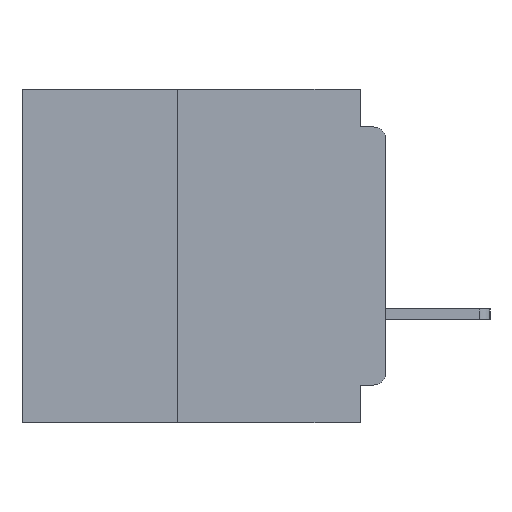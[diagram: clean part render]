
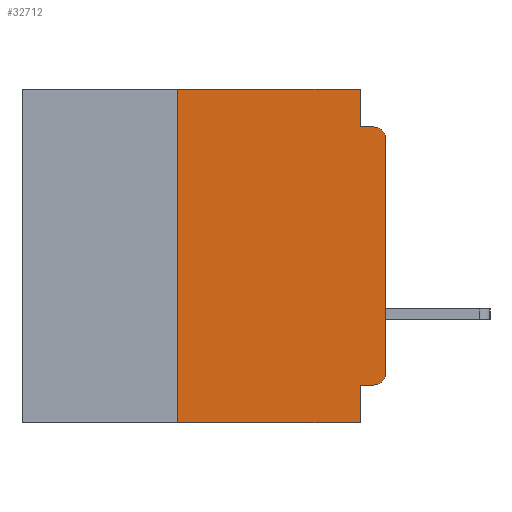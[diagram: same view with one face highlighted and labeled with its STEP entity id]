
A CAD part, left-side view. The second image highlights one B-rep face of the part: STEP entity #32712.
In plain terms, the highlighted planar face has unit normal (-1, 0, 0).
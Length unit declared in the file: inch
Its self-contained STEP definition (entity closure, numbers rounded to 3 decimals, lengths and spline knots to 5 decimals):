
#742 = LINE ( 'NONE', #29667, #42901 ) ;
#1941 = VECTOR ( 'NONE', #19512, 39.37008 ) ;
#3548 = DIRECTION ( 'NONE',  ( 0., 1., 0. ) ) ;
#6197 = ORIENTED_EDGE ( 'NONE', *, *, #39112, .T. ) ;
#7987 = AXIS2_PLACEMENT_3D ( 'NONE', #17794, #46150, #21936 ) ;
#8989 = CARTESIAN_POINT ( 'NONE',  ( 0., 0., 0. ) ) ;
#9048 = CARTESIAN_POINT ( 'NONE',  ( 0., 0.031, -0.045 ) ) ;
#9254 = DIRECTION ( 'NONE',  ( 1., 0., 0. ) ) ;
#9734 = VERTEX_POINT ( 'NONE', #20476 ) ;
#10801 = AXIS2_PLACEMENT_3D ( 'NONE', #39432, #15084, #43482 ) ;
#11377 = VERTEX_POINT ( 'NONE', #9048 ) ;
#12565 = LINE ( 'NONE', #51588, #51837 ) ;
#13140 = VECTOR ( 'NONE', #46904, 39.37008 ) ;
#13155 = DIRECTION ( 'NONE',  ( 0., 0., 1. ) ) ;
#13230 = PLANE ( 'NONE',  #24703 ) ;
#13568 = VERTEX_POINT ( 'NONE', #38144 ) ;
#13709 = ORIENTED_EDGE ( 'NONE', *, *, #46031, .F. ) ;
#14898 = VERTEX_POINT ( 'NONE', #47126 ) ;
#15084 = DIRECTION ( 'NONE',  ( -1., 0., 0. ) ) ;
#15386 = CARTESIAN_POINT ( 'NONE',  ( 0., 0.437, -0.4 ) ) ;
#15509 = EDGE_CURVE ( 'NONE', #13568, #34207, #34827, .T. ) ;
#15622 = EDGE_CURVE ( 'NONE', #34207, #42120, #27241, .T. ) ;
#15964 = CIRCLE ( 'NONE', #7987, 0.015 ) ;
#16896 = CARTESIAN_POINT ( 'NONE',  ( 0., 0.031, -0.4 ) ) ;
#17794 = CARTESIAN_POINT ( 'NONE',  ( 0., 0.015, -0.34 ) ) ;
#17914 = EDGE_CURVE ( 'NONE', #13568, #43147, #23846, .T. ) ;
#18343 = CARTESIAN_POINT ( 'NONE',  ( 0., 0.031, -0.4 ) ) ;
#18580 = CARTESIAN_POINT ( 'NONE',  ( 0., 0.25, -0.4 ) ) ;
#18946 = EDGE_CURVE ( 'NONE', #38450, #43147, #40191, .T. ) ;
#19512 = DIRECTION ( 'NONE',  ( 0., -1., 0. ) ) ;
#20476 = CARTESIAN_POINT ( 'NONE',  ( 0., 0., -0.06 ) ) ;
#21034 = DIRECTION ( 'NONE',  ( 0., 0., -1. ) ) ;
#21538 = FACE_OUTER_BOUND ( 'NONE', #50011, .T. ) ;
#21640 = ORIENTED_EDGE ( 'NONE', *, *, #18946, .F. ) ;
#21936 = DIRECTION ( 'NONE',  ( 0., 0., -1. ) ) ;
#22992 = VECTOR ( 'NONE', #3548, 39.37008 ) ;
#23239 = EDGE_CURVE ( 'NONE', #11377, #14898, #12565, .T. ) ;
#23354 = ORIENTED_EDGE ( 'NONE', *, *, #24759, .F. ) ;
#23600 = CARTESIAN_POINT ( 'NONE',  ( 0., 0.437, 0. ) ) ;
#23846 = LINE ( 'NONE', #15386, #1941 ) ;
#24703 = AXIS2_PLACEMENT_3D ( 'NONE', #25595, #9254, #37783 ) ;
#24759 = EDGE_CURVE ( 'NONE', #42120, #11377, #742, .T. ) ;
#25595 = CARTESIAN_POINT ( 'NONE',  ( 0., 0.437, 0. ) ) ;
#26967 = VERTEX_POINT ( 'NONE', #52429 ) ;
#27241 = LINE ( 'NONE', #23600, #47369 ) ;
#27694 = DIRECTION ( 'NONE',  ( 0., -1., 0. ) ) ;
#28161 = EDGE_CURVE ( 'NONE', #9734, #14898, #46636, .T. ) ;
#29428 = CARTESIAN_POINT ( 'NONE',  ( 0., 0.031, -0.355 ) ) ;
#29667 = CARTESIAN_POINT ( 'NONE',  ( 0., 0.031, 0. ) ) ;
#31478 = ORIENTED_EDGE ( 'NONE', *, *, #17914, .T. ) ;
#31873 = CARTESIAN_POINT ( 'NONE',  ( 0., 0.031, 0. ) ) ;
#32712 = ADVANCED_FACE ( 'NONE', ( #21538 ), #13230, .F. ) ;
#33252 = ORIENTED_EDGE ( 'NONE', *, *, #23239, .F. ) ;
#33271 = VERTEX_POINT ( 'NONE', #50882 ) ;
#34207 = VERTEX_POINT ( 'NONE', #41523 ) ;
#34827 = LINE ( 'NONE', #18580, #13140 ) ;
#35737 = VECTOR ( 'NONE', #13155, 39.37008 ) ;
#36288 = CARTESIAN_POINT ( 'NONE',  ( 0., 0., -0.355 ) ) ;
#36324 = LINE ( 'NONE', #36288, #22992 ) ;
#36413 = VECTOR ( 'NONE', #21034, 39.37008 ) ;
#37783 = DIRECTION ( 'NONE',  ( 0., 0., -1. ) ) ;
#38144 = CARTESIAN_POINT ( 'NONE',  ( 0., 0.25, -0.4 ) ) ;
#38450 = VERTEX_POINT ( 'NONE', #29428 ) ;
#39112 = EDGE_CURVE ( 'NONE', #26967, #9734, #46394, .T. ) ;
#39432 = CARTESIAN_POINT ( 'NONE',  ( 0., 0.015, -0.06 ) ) ;
#40191 = LINE ( 'NONE', #16896, #36413 ) ;
#40944 = ORIENTED_EDGE ( 'NONE', *, *, #45642, .T. ) ;
#41277 = ORIENTED_EDGE ( 'NONE', *, *, #15622, .F. ) ;
#41523 = CARTESIAN_POINT ( 'NONE',  ( 0., 0.25, 0. ) ) ;
#42120 = VERTEX_POINT ( 'NONE', #31873 ) ;
#42901 = VECTOR ( 'NONE', #45627, 39.37008 ) ;
#43147 = VERTEX_POINT ( 'NONE', #18343 ) ;
#43482 = DIRECTION ( 'NONE',  ( 0., 0., -1. ) ) ;
#45627 = DIRECTION ( 'NONE',  ( 0., 0., -1. ) ) ;
#45642 = EDGE_CURVE ( 'NONE', #33271, #26967, #15964, .T. ) ;
#46031 = EDGE_CURVE ( 'NONE', #33271, #38450, #36324, .T. ) ;
#46150 = DIRECTION ( 'NONE',  ( -1., 0., 0. ) ) ;
#46394 = LINE ( 'NONE', #8989, #35737 ) ;
#46636 = CIRCLE ( 'NONE', #10801, 0.015 ) ;
#46904 = DIRECTION ( 'NONE',  ( 0., 0., 1. ) ) ;
#47126 = CARTESIAN_POINT ( 'NONE',  ( 0., 0.015, -0.045 ) ) ;
#47369 = VECTOR ( 'NONE', #47764, 39.37008 ) ;
#47764 = DIRECTION ( 'NONE',  ( 0., -1., 0. ) ) ;
#47807 = ORIENTED_EDGE ( 'NONE', *, *, #28161, .T. ) ;
#50011 = EDGE_LOOP ( 'NONE', ( #6197, #47807, #33252, #23354, #41277, #50135, #31478, #21640, #13709, #40944 ) ) ;
#50135 = ORIENTED_EDGE ( 'NONE', *, *, #15509, .F. ) ;
#50882 = CARTESIAN_POINT ( 'NONE',  ( 0., 0.015, -0.355 ) ) ;
#51588 = CARTESIAN_POINT ( 'NONE',  ( 0., 0., -0.045 ) ) ;
#51837 = VECTOR ( 'NONE', #27694, 39.37008 ) ;
#52429 = CARTESIAN_POINT ( 'NONE',  ( 0., 0., -0.34 ) ) ;
